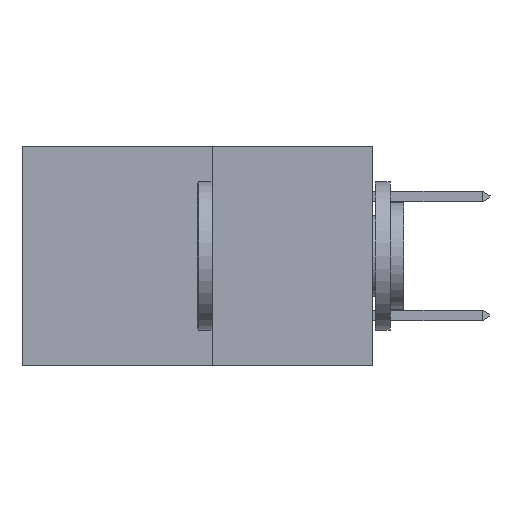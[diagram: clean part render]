
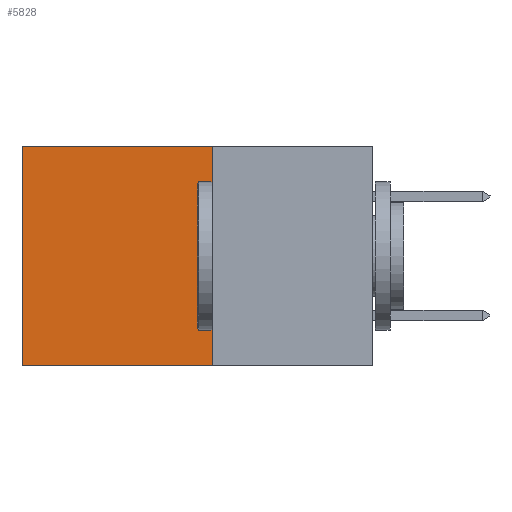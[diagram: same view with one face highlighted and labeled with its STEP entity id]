
A CAD part, left-side view. The second image highlights one B-rep face of the part: STEP entity #5828.
In plain terms, the highlighted planar face has unit normal (-1, 0, 0).
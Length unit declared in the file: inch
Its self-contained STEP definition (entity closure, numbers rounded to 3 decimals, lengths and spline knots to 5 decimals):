
#522 = VECTOR ( 'NONE', #1561, 39.37008 ) ;
#843 = DIRECTION ( 'NONE',  ( 0., 1., 0. ) ) ;
#1280 = EDGE_CURVE ( 'NONE', #6869, #6856, #4322, .T. ) ;
#1561 = DIRECTION ( 'NONE',  ( 0., 0., -1. ) ) ;
#2247 = CARTESIAN_POINT ( 'NONE',  ( 0.277, 0.27, -0.37 ) ) ;
#2818 = VECTOR ( 'NONE', #15660, 39.37008 ) ;
#3459 = LINE ( 'NONE', #10213, #522 ) ;
#4322 = LINE ( 'NONE', #2247, #11984 ) ;
#4645 = FACE_OUTER_BOUND ( 'NONE', #11226, .T. ) ;
#5506 = EDGE_CURVE ( 'NONE', #11035, #6869, #10541, .T. ) ;
#5828 = ADVANCED_FACE ( 'NONE', ( #4645 ), #12604, .F. ) ;
#6190 = ORIENTED_EDGE ( 'NONE', *, *, #5506, .F. ) ;
#6856 = VERTEX_POINT ( 'NONE', #9434 ) ;
#6869 = VERTEX_POINT ( 'NONE', #8116 ) ;
#8116 = CARTESIAN_POINT ( 'NONE',  ( 0.277, 0.27, -0.37 ) ) ;
#9145 = ORIENTED_EDGE ( 'NONE', *, *, #1280, .F. ) ;
#9434 = CARTESIAN_POINT ( 'NONE',  ( 0.277, 0.59, -0.37 ) ) ;
#9505 = CARTESIAN_POINT ( 'NONE',  ( 0.277, 0.27, 0. ) ) ;
#9537 = VERTEX_POINT ( 'NONE', #17914 ) ;
#9983 = LINE ( 'NONE', #9505, #14841 ) ;
#10213 = CARTESIAN_POINT ( 'NONE',  ( 0.277, 0.59, -0.37 ) ) ;
#10507 = ORIENTED_EDGE ( 'NONE', *, *, #18764, .T. ) ;
#10541 = LINE ( 'NONE', #14418, #2818 ) ;
#11035 = VERTEX_POINT ( 'NONE', #16661 ) ;
#11226 = EDGE_LOOP ( 'NONE', ( #12526, #9145, #6190, #10507 ) ) ;
#11984 = VECTOR ( 'NONE', #15219, 39.37008 ) ;
#12526 = ORIENTED_EDGE ( 'NONE', *, *, #17568, .T. ) ;
#12604 = PLANE ( 'NONE',  #15742 ) ;
#12636 = CARTESIAN_POINT ( 'NONE',  ( 0.277, 0.27, -0.37 ) ) ;
#12655 = DIRECTION ( 'NONE',  ( 1., 0., 0. ) ) ;
#12778 = DIRECTION ( 'NONE',  ( 0., 0., -1. ) ) ;
#14418 = CARTESIAN_POINT ( 'NONE',  ( 0.277, 0.27, -0.37 ) ) ;
#14841 = VECTOR ( 'NONE', #843, 39.37008 ) ;
#15219 = DIRECTION ( 'NONE',  ( 0., 1., 0. ) ) ;
#15660 = DIRECTION ( 'NONE',  ( 0., 0., -1. ) ) ;
#15742 = AXIS2_PLACEMENT_3D ( 'NONE', #12636, #12655, #12778 ) ;
#16661 = CARTESIAN_POINT ( 'NONE',  ( 0.277, 0.27, 0. ) ) ;
#17568 = EDGE_CURVE ( 'NONE', #9537, #6856, #3459, .T. ) ;
#17914 = CARTESIAN_POINT ( 'NONE',  ( 0.277, 0.59, 0. ) ) ;
#18764 = EDGE_CURVE ( 'NONE', #11035, #9537, #9983, .T. ) ;
